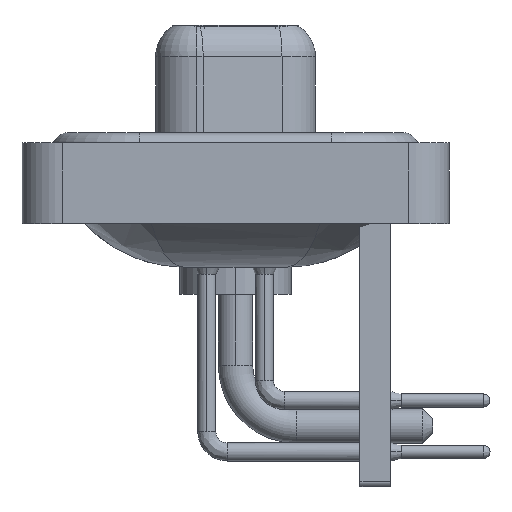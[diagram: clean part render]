
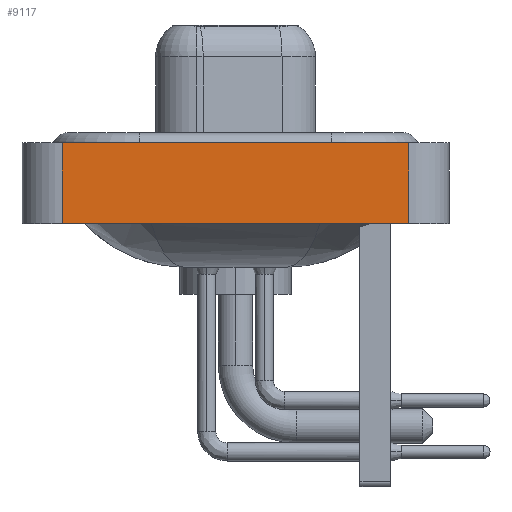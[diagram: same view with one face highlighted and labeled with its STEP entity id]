
A CAD part, left-side view. The second image highlights one B-rep face of the part: STEP entity #9117.
In plain terms, the highlighted planar face has unit normal (-1, 0, 0).
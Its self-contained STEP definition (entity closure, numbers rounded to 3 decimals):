
#780 = DIRECTION ( 'NONE',  ( 0., -1., 0. ) ) ;
#1473 = VECTOR ( 'NONE', #12981, 1000. ) ;
#1584 = CARTESIAN_POINT ( 'NONE',  ( -7.25, -8.55, -3.6 ) ) ;
#1658 = CARTESIAN_POINT ( 'NONE',  ( -7.25, -8.55, 0.4 ) ) ;
#1663 = VERTEX_POINT ( 'NONE', #2383 ) ;
#2383 = CARTESIAN_POINT ( 'NONE',  ( -7.25, -8.55, -3.6 ) ) ;
#3787 = EDGE_CURVE ( 'NONE', #10585, #18009, #5618, .T. ) ;
#3913 = VECTOR ( 'NONE', #780, 1000. ) ;
#4874 = LINE ( 'NONE', #1584, #1473 ) ;
#5417 = VERTEX_POINT ( 'NONE', #1658 ) ;
#5618 = LINE ( 'NONE', #13201, #17913 ) ;
#6082 = CARTESIAN_POINT ( 'NONE',  ( -7.25, -8.55, -3.6 ) ) ;
#7563 = PLANE ( 'NONE',  #16878 ) ;
#7790 = CARTESIAN_POINT ( 'NONE',  ( -7.25, 8.55, -3.6 ) ) ;
#7872 = FACE_OUTER_BOUND ( 'NONE', #20252, .T. ) ;
#8075 = LINE ( 'NONE', #20790, #15888 ) ;
#9007 = LINE ( 'NONE', #15191, #3913 ) ;
#9117 = ADVANCED_FACE ( 'NONE', ( #7872 ), #7563, .T. ) ;
#9261 = EDGE_CURVE ( 'NONE', #10585, #1663, #8075, .T. ) ;
#9590 = ORIENTED_EDGE ( 'NONE', *, *, #10159, .T. ) ;
#10159 = EDGE_CURVE ( 'NONE', #1663, #5417, #4874, .T. ) ;
#10585 = VERTEX_POINT ( 'NONE', #7790 ) ;
#11339 = DIRECTION ( 'NONE',  ( 0., -1., 0. ) ) ;
#12047 = DIRECTION ( 'NONE',  ( 0., 0., 1. ) ) ;
#12114 = CARTESIAN_POINT ( 'NONE',  ( -7.25, 8.55, 0.4 ) ) ;
#12981 = DIRECTION ( 'NONE',  ( 0., 0., 1. ) ) ;
#13201 = CARTESIAN_POINT ( 'NONE',  ( -7.25, 8.55, -3.6 ) ) ;
#14182 = DIRECTION ( 'NONE',  ( 0., 0., 1. ) ) ;
#14212 = ORIENTED_EDGE ( 'NONE', *, *, #9261, .T. ) ;
#15191 = CARTESIAN_POINT ( 'NONE',  ( -7.25, -8.55, 0.4 ) ) ;
#15888 = VECTOR ( 'NONE', #11339, 1000. ) ;
#16878 = AXIS2_PLACEMENT_3D ( 'NONE', #6082, #18905, #14182 ) ;
#17913 = VECTOR ( 'NONE', #12047, 1000. ) ;
#18009 = VERTEX_POINT ( 'NONE', #12114 ) ;
#18482 = ORIENTED_EDGE ( 'NONE', *, *, #3787, .F. ) ;
#18748 = EDGE_CURVE ( 'NONE', #18009, #5417, #9007, .T. ) ;
#18905 = DIRECTION ( 'NONE',  ( -1., 0., 0. ) ) ;
#19577 = ORIENTED_EDGE ( 'NONE', *, *, #18748, .F. ) ;
#20252 = EDGE_LOOP ( 'NONE', ( #9590, #19577, #18482, #14212 ) ) ;
#20790 = CARTESIAN_POINT ( 'NONE',  ( -7.25, -8.55, -3.6 ) ) ;
